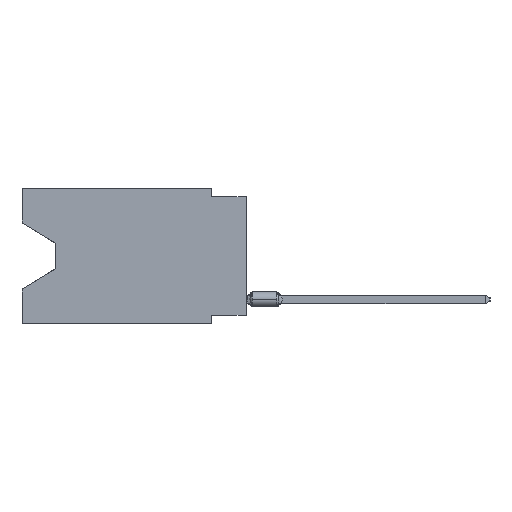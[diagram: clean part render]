
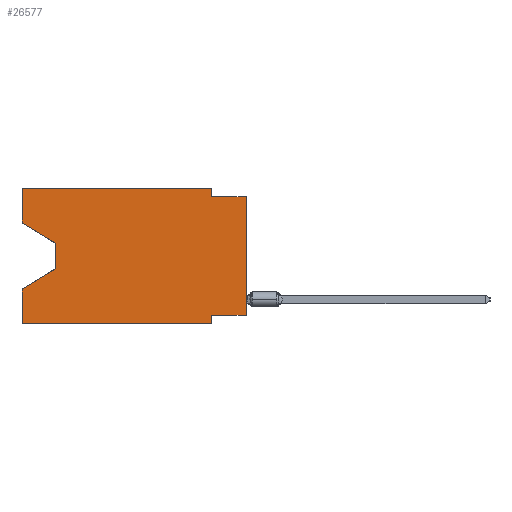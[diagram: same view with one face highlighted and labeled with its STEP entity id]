
A CAD part, left-side view. The second image highlights one B-rep face of the part: STEP entity #26577.
In plain terms, the highlighted planar face has unit normal (-1, 0, 0).
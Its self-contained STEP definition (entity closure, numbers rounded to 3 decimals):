
#389 = DIRECTION ( 'NONE',  ( 1., 0., 0. ) ) ;
#668 = CARTESIAN_POINT ( 'NONE',  ( 0., 0., -9.271 ) ) ;
#930 = LINE ( 'NONE', #32136, #32503 ) ;
#991 = LINE ( 'NONE', #8931, #8164 ) ;
#1092 = CARTESIAN_POINT ( 'NONE',  ( 0., 16.383, -9.906 ) ) ;
#1285 = DIRECTION ( 'NONE',  ( 0., 0., -1. ) ) ;
#2337 = LINE ( 'NONE', #12628, #32366 ) ;
#2363 = VERTEX_POINT ( 'NONE', #1092 ) ;
#2468 = VERTEX_POINT ( 'NONE', #19830 ) ;
#2850 = AXIS2_PLACEMENT_3D ( 'NONE', #28928, #389, #10536 ) ;
#3374 = LINE ( 'NONE', #668, #18589 ) ;
#3440 = VECTOR ( 'NONE', #32552, 1000. ) ;
#4292 = DIRECTION ( 'NONE',  ( 0., -0.855, -0.519 ) ) ;
#4317 = DIRECTION ( 'NONE',  ( 0., 0., 1. ) ) ;
#4563 = ORIENTED_EDGE ( 'NONE', *, *, #33097, .F. ) ;
#4854 = ORIENTED_EDGE ( 'NONE', *, *, #8102, .T. ) ;
#5627 = FACE_OUTER_BOUND ( 'NONE', #19714, .T. ) ;
#5668 = VERTEX_POINT ( 'NONE', #14659 ) ;
#6270 = CARTESIAN_POINT ( 'NONE',  ( 0., 0., -0.635 ) ) ;
#6436 = LINE ( 'NONE', #23675, #14542 ) ;
#6453 = LINE ( 'NONE', #16263, #12379 ) ;
#6563 = CARTESIAN_POINT ( 'NONE',  ( 0., 16.383, -9.906 ) ) ;
#7090 = DIRECTION ( 'NONE',  ( 0., -1., 0. ) ) ;
#7858 = ORIENTED_EDGE ( 'NONE', *, *, #31503, .T. ) ;
#8102 = EDGE_CURVE ( 'NONE', #2468, #25521, #20225, .T. ) ;
#8164 = VECTOR ( 'NONE', #11279, 1000. ) ;
#8931 = CARTESIAN_POINT ( 'NONE',  ( 0., 16.383, 0. ) ) ;
#9282 = VECTOR ( 'NONE', #1285, 1000. ) ;
#9385 = VERTEX_POINT ( 'NONE', #18861 ) ;
#9908 = CARTESIAN_POINT ( 'NONE',  ( 0., 13.97, -4.013 ) ) ;
#10103 = VERTEX_POINT ( 'NONE', #25232 ) ;
#10536 = DIRECTION ( 'NONE',  ( 0., 0., -1. ) ) ;
#11279 = DIRECTION ( 'NONE',  ( 0., 0., 1. ) ) ;
#12301 = EDGE_CURVE ( 'NONE', #25685, #27707, #6453, .T. ) ;
#12307 = DIRECTION ( 'NONE',  ( 0., 0., 1. ) ) ;
#12379 = VECTOR ( 'NONE', #7090, 1000. ) ;
#12476 = VECTOR ( 'NONE', #29239, 1000. ) ;
#12628 = CARTESIAN_POINT ( 'NONE',  ( 0., 2.54, 0. ) ) ;
#12657 = LINE ( 'NONE', #28008, #19453 ) ;
#12806 = EDGE_CURVE ( 'NONE', #27707, #20252, #2337, .T. ) ;
#13074 = EDGE_CURVE ( 'NONE', #2363, #25521, #27451, .T. ) ;
#13713 = LINE ( 'NONE', #6270, #12476 ) ;
#14012 = LINE ( 'NONE', #6563, #3440 ) ;
#14542 = VECTOR ( 'NONE', #31751, 1000. ) ;
#14659 = CARTESIAN_POINT ( 'NONE',  ( 0., 16.383, -2.546 ) ) ;
#16263 = CARTESIAN_POINT ( 'NONE',  ( 0., 16.383, 0. ) ) ;
#17174 = ORIENTED_EDGE ( 'NONE', *, *, #28638, .T. ) ;
#17451 = CARTESIAN_POINT ( 'NONE',  ( 0., 16.383, -7.36 ) ) ;
#17672 = ORIENTED_EDGE ( 'NONE', *, *, #12806, .F. ) ;
#17724 = EDGE_CURVE ( 'NONE', #5668, #25685, #991, .T. ) ;
#18589 = VECTOR ( 'NONE', #33112, 1000. ) ;
#18861 = CARTESIAN_POINT ( 'NONE',  ( 0., 2.54, -9.906 ) ) ;
#19402 = ORIENTED_EDGE ( 'NONE', *, *, #17724, .F. ) ;
#19453 = VECTOR ( 'NONE', #12307, 1000. ) ;
#19488 = CARTESIAN_POINT ( 'NONE',  ( 0., 2.54, -9.906 ) ) ;
#19572 = EDGE_CURVE ( 'NONE', #2363, #9385, #14012, .T. ) ;
#19714 = EDGE_LOOP ( 'NONE', ( #7858, #17174, #4854, #31066, #31577, #32483, #4563, #26864, #28654, #17672, #22985, #19402 ) ) ;
#19830 = CARTESIAN_POINT ( 'NONE',  ( 0., 13.97, -5.893 ) ) ;
#20225 = LINE ( 'NONE', #25459, #24523 ) ;
#20252 = VERTEX_POINT ( 'NONE', #31705 ) ;
#20655 = PLANE ( 'NONE',  #2850 ) ;
#20703 = CARTESIAN_POINT ( 'NONE',  ( 0., 2.54, 0. ) ) ;
#21115 = CARTESIAN_POINT ( 'NONE',  ( 0., 2.54, -9.271 ) ) ;
#21662 = CARTESIAN_POINT ( 'NONE',  ( 0., 16.383, 0. ) ) ;
#22985 = ORIENTED_EDGE ( 'NONE', *, *, #12301, .F. ) ;
#23242 = EDGE_CURVE ( 'NONE', #20252, #10103, #13713, .T. ) ;
#23258 = VECTOR ( 'NONE', #4317, 1000. ) ;
#23675 = CARTESIAN_POINT ( 'NONE',  ( 0., 13.97, -4.013 ) ) ;
#24332 = VERTEX_POINT ( 'NONE', #21115 ) ;
#24422 = LINE ( 'NONE', #19488, #9282 ) ;
#24523 = VECTOR ( 'NONE', #25969, 1000. ) ;
#24594 = EDGE_CURVE ( 'NONE', #25896, #10103, #12657, .T. ) ;
#25232 = CARTESIAN_POINT ( 'NONE',  ( 0., 0., -0.635 ) ) ;
#25310 = EDGE_CURVE ( 'NONE', #24332, #9385, #24422, .T. ) ;
#25459 = CARTESIAN_POINT ( 'NONE',  ( 0., 13.97, -5.893 ) ) ;
#25521 = VERTEX_POINT ( 'NONE', #17451 ) ;
#25685 = VERTEX_POINT ( 'NONE', #21662 ) ;
#25896 = VERTEX_POINT ( 'NONE', #26433 ) ;
#25969 = DIRECTION ( 'NONE',  ( 0., 0.855, -0.519 ) ) ;
#26433 = CARTESIAN_POINT ( 'NONE',  ( 0., 0., -9.271 ) ) ;
#26577 = ADVANCED_FACE ( 'NONE', ( #5627 ), #20655, .F. ) ;
#26864 = ORIENTED_EDGE ( 'NONE', *, *, #24594, .T. ) ;
#27451 = LINE ( 'NONE', #30125, #23258 ) ;
#27707 = VERTEX_POINT ( 'NONE', #20703 ) ;
#28008 = CARTESIAN_POINT ( 'NONE',  ( 0., 0., 0. ) ) ;
#28638 = EDGE_CURVE ( 'NONE', #29731, #2468, #6436, .T. ) ;
#28654 = ORIENTED_EDGE ( 'NONE', *, *, #23242, .F. ) ;
#28928 = CARTESIAN_POINT ( 'NONE',  ( 0., 16.383, 0. ) ) ;
#29239 = DIRECTION ( 'NONE',  ( 0., -1., 0. ) ) ;
#29731 = VERTEX_POINT ( 'NONE', #9908 ) ;
#30125 = CARTESIAN_POINT ( 'NONE',  ( 0., 16.383, 0. ) ) ;
#30165 = DIRECTION ( 'NONE',  ( 0., 0., -1. ) ) ;
#31066 = ORIENTED_EDGE ( 'NONE', *, *, #13074, .F. ) ;
#31503 = EDGE_CURVE ( 'NONE', #5668, #29731, #930, .T. ) ;
#31577 = ORIENTED_EDGE ( 'NONE', *, *, #19572, .T. ) ;
#31705 = CARTESIAN_POINT ( 'NONE',  ( 0., 2.54, -0.635 ) ) ;
#31751 = DIRECTION ( 'NONE',  ( 0., 0., -1. ) ) ;
#32136 = CARTESIAN_POINT ( 'NONE',  ( 0., 16.383, -2.546 ) ) ;
#32366 = VECTOR ( 'NONE', #30165, 1000. ) ;
#32483 = ORIENTED_EDGE ( 'NONE', *, *, #25310, .F. ) ;
#32503 = VECTOR ( 'NONE', #4292, 1000. ) ;
#32552 = DIRECTION ( 'NONE',  ( 0., -1., 0. ) ) ;
#33097 = EDGE_CURVE ( 'NONE', #25896, #24332, #3374, .T. ) ;
#33112 = DIRECTION ( 'NONE',  ( 0., 1., 0. ) ) ;
